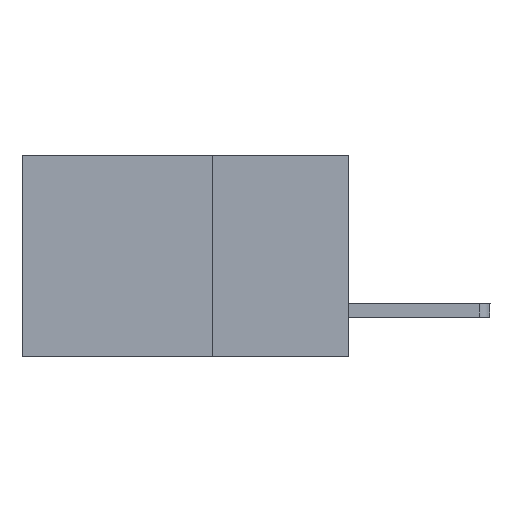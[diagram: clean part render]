
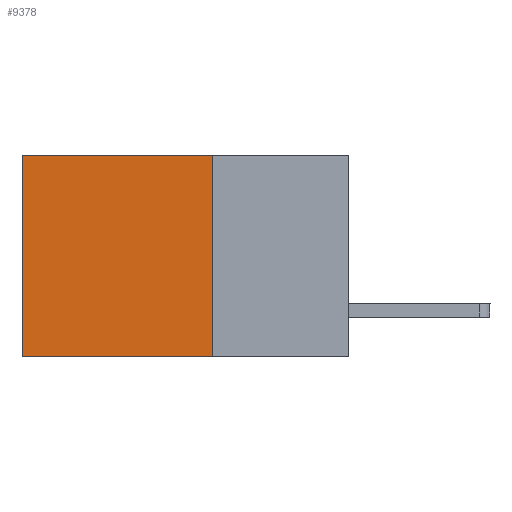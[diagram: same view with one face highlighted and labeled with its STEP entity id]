
A CAD part, left-side view. The second image highlights one B-rep face of the part: STEP entity #9378.
In plain terms, the highlighted planar face has unit normal (-1, 0, 0).
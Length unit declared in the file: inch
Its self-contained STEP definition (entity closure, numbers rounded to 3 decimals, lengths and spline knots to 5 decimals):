
#7 = CARTESIAN_POINT ( 'NONE',  ( 0.2615, 0.6, 0. ) ) ;
#124 = VERTEX_POINT ( 'NONE', #1229 ) ;
#563 = DIRECTION ( 'NONE',  ( 0., 1., 0. ) ) ;
#1229 = CARTESIAN_POINT ( 'NONE',  ( 0.2615, 0.25, 0. ) ) ;
#1429 = VERTEX_POINT ( 'NONE', #7 ) ;
#1652 = EDGE_LOOP ( 'NONE', ( #9833, #3881, #5655, #6737 ) ) ;
#1783 = PLANE ( 'NONE',  #2335 ) ;
#1839 = DIRECTION ( 'NONE',  ( 0., 0., -1. ) ) ;
#2277 = EDGE_CURVE ( 'NONE', #124, #1429, #9856, .T. ) ;
#2335 = AXIS2_PLACEMENT_3D ( 'NONE', #8207, #4114, #1839 ) ;
#2397 = CARTESIAN_POINT ( 'NONE',  ( 0.2615, 0.6, -0.37 ) ) ;
#2434 = CARTESIAN_POINT ( 'NONE',  ( 0.2615, 0.25, 0. ) ) ;
#2443 = CARTESIAN_POINT ( 'NONE',  ( 0.2615, 0.6, -0.37 ) ) ;
#2601 = CARTESIAN_POINT ( 'NONE',  ( 0.2615, 0.25, -0.37 ) ) ;
#2925 = EDGE_CURVE ( 'NONE', #1429, #7462, #8770, .T. ) ;
#3424 = DIRECTION ( 'NONE',  ( 0., 1., 0. ) ) ;
#3881 = ORIENTED_EDGE ( 'NONE', *, *, #4096, .F. ) ;
#4096 = EDGE_CURVE ( 'NONE', #5075, #7462, #10377, .T. ) ;
#4114 = DIRECTION ( 'NONE',  ( 1., 0., 0. ) ) ;
#4464 = EDGE_CURVE ( 'NONE', #124, #5075, #5450, .T. ) ;
#4571 = DIRECTION ( 'NONE',  ( 0., 0., -1. ) ) ;
#5075 = VERTEX_POINT ( 'NONE', #2601 ) ;
#5450 = LINE ( 'NONE', #9520, #7025 ) ;
#5655 = ORIENTED_EDGE ( 'NONE', *, *, #4464, .F. ) ;
#5672 = FACE_OUTER_BOUND ( 'NONE', #1652, .T. ) ;
#6415 = VECTOR ( 'NONE', #3424, 39.37008 ) ;
#6737 = ORIENTED_EDGE ( 'NONE', *, *, #2277, .T. ) ;
#7025 = VECTOR ( 'NONE', #4571, 39.37008 ) ;
#7429 = VECTOR ( 'NONE', #563, 39.37008 ) ;
#7462 = VERTEX_POINT ( 'NONE', #2443 ) ;
#7611 = VECTOR ( 'NONE', #8723, 39.37008 ) ;
#7981 = CARTESIAN_POINT ( 'NONE',  ( 0.2615, 0.25, -0.37 ) ) ;
#8207 = CARTESIAN_POINT ( 'NONE',  ( 0.2615, 0.25, -0.37 ) ) ;
#8723 = DIRECTION ( 'NONE',  ( 0., 0., -1. ) ) ;
#8770 = LINE ( 'NONE', #2397, #7611 ) ;
#9378 = ADVANCED_FACE ( 'NONE', ( #5672 ), #1783, .F. ) ;
#9520 = CARTESIAN_POINT ( 'NONE',  ( 0.2615, 0.25, -0.37 ) ) ;
#9833 = ORIENTED_EDGE ( 'NONE', *, *, #2925, .T. ) ;
#9856 = LINE ( 'NONE', #2434, #6415 ) ;
#10377 = LINE ( 'NONE', #7981, #7429 ) ;
